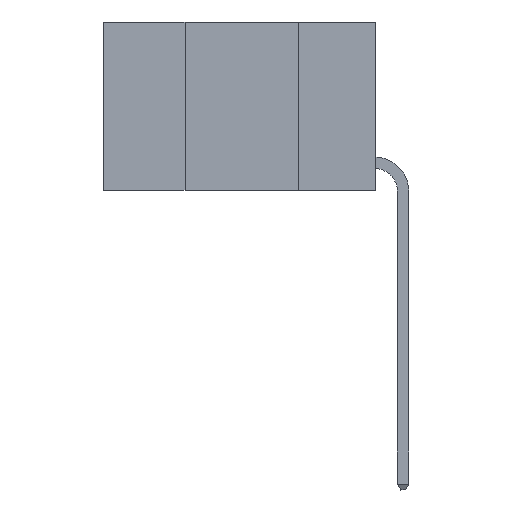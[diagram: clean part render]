
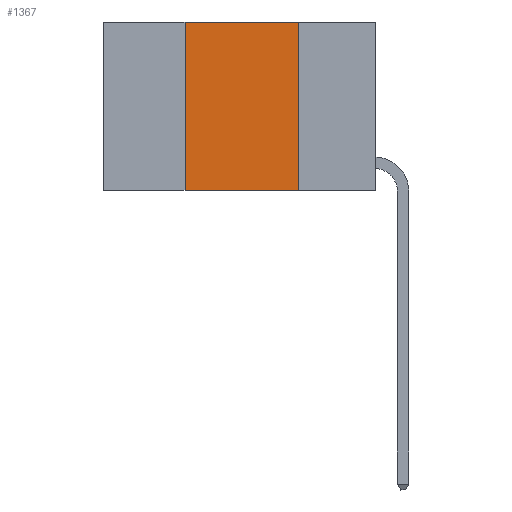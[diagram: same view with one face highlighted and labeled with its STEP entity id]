
A CAD part, left-side view. The second image highlights one B-rep face of the part: STEP entity #1367.
In plain terms, the highlighted planar face has unit normal (-1, 0, 0).
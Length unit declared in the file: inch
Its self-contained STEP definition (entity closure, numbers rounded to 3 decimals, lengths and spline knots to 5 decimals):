
#15 = VECTOR ( 'NONE', #6879, 39.37008 ) ;
#139 = CARTESIAN_POINT ( 'NONE',  ( 0., 0.17, 0. ) ) ;
#154 = VERTEX_POINT ( 'NONE', #7623 ) ;
#467 = ORIENTED_EDGE ( 'NONE', *, *, #5842, .F. ) ;
#640 = ORIENTED_EDGE ( 'NONE', *, *, #5004, .T. ) ;
#889 = DIRECTION ( 'NONE',  ( 0., 0., 1. ) ) ;
#1282 = FACE_OUTER_BOUND ( 'NONE', #5051, .T. ) ;
#1367 = ADVANCED_FACE ( 'NONE', ( #1282 ), #4138, .F. ) ;
#1620 = AXIS2_PLACEMENT_3D ( 'NONE', #2086, #5779, #7791 ) ;
#1645 = DIRECTION ( 'NONE',  ( 0., -1., 0. ) ) ;
#1860 = VERTEX_POINT ( 'NONE', #139 ) ;
#1991 = VERTEX_POINT ( 'NONE', #2600 ) ;
#2086 = CARTESIAN_POINT ( 'NONE',  ( 0., 0.6, 0. ) ) ;
#2589 = EDGE_CURVE ( 'NONE', #1991, #1860, #7051, .T. ) ;
#2600 = CARTESIAN_POINT ( 'NONE',  ( 0., 0.42, 0. ) ) ;
#2626 = EDGE_CURVE ( 'NONE', #6197, #1991, #4477, .T. ) ;
#2688 = VECTOR ( 'NONE', #889, 39.37008 ) ;
#4138 = PLANE ( 'NONE',  #1620 ) ;
#4477 = LINE ( 'NONE', #7900, #2688 ) ;
#4699 = ORIENTED_EDGE ( 'NONE', *, *, #2589, .F. ) ;
#4845 = LINE ( 'NONE', #5968, #15 ) ;
#5004 = EDGE_CURVE ( 'NONE', #6197, #154, #4845, .T. ) ;
#5051 = EDGE_LOOP ( 'NONE', ( #467, #4699, #6547, #640 ) ) ;
#5667 = CARTESIAN_POINT ( 'NONE',  ( 0., 0.6, 0. ) ) ;
#5779 = DIRECTION ( 'NONE',  ( 1., 0., 0. ) ) ;
#5842 = EDGE_CURVE ( 'NONE', #1860, #154, #7411, .T. ) ;
#5968 = CARTESIAN_POINT ( 'NONE',  ( 0., 0.6, -0.37 ) ) ;
#6197 = VERTEX_POINT ( 'NONE', #7693 ) ;
#6415 = VECTOR ( 'NONE', #6543, 39.37008 ) ;
#6543 = DIRECTION ( 'NONE',  ( 0., 0., -1. ) ) ;
#6547 = ORIENTED_EDGE ( 'NONE', *, *, #2626, .F. ) ;
#6637 = CARTESIAN_POINT ( 'NONE',  ( 0., 0.17, 0. ) ) ;
#6879 = DIRECTION ( 'NONE',  ( 0., -1., 0. ) ) ;
#7051 = LINE ( 'NONE', #5667, #7837 ) ;
#7411 = LINE ( 'NONE', #6637, #6415 ) ;
#7623 = CARTESIAN_POINT ( 'NONE',  ( 0., 0.17, -0.37 ) ) ;
#7693 = CARTESIAN_POINT ( 'NONE',  ( 0., 0.42, -0.37 ) ) ;
#7791 = DIRECTION ( 'NONE',  ( 0., 0., -1. ) ) ;
#7837 = VECTOR ( 'NONE', #1645, 39.37008 ) ;
#7900 = CARTESIAN_POINT ( 'NONE',  ( 0., 0.42, 0. ) ) ;
